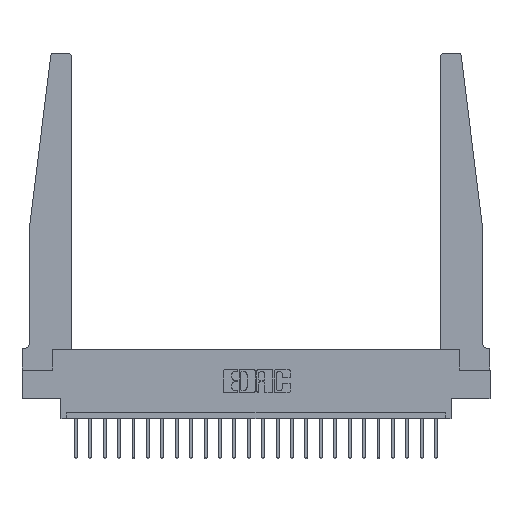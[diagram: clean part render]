
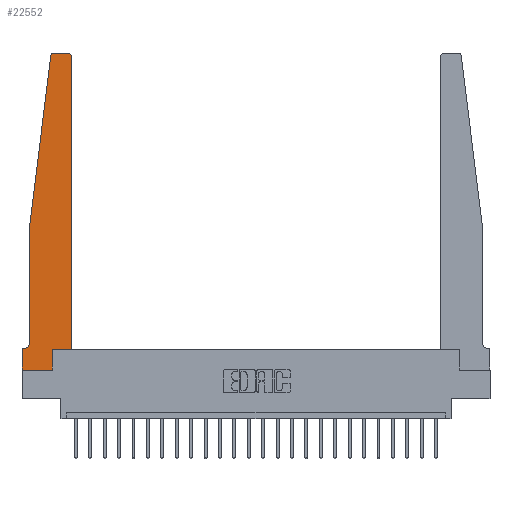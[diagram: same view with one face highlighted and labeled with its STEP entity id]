
A CAD part, top view. The second image highlights one B-rep face of the part: STEP entity #22552.
In plain terms, the highlighted planar face has unit normal (0, 0, 1).
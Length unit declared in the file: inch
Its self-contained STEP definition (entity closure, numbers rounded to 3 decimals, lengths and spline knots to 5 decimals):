
#285 = EDGE_CURVE ( 'NONE', #22686, #6802, #12120, .T. ) ;
#402 = VECTOR ( 'NONE', #20347, 39.37008 ) ;
#413 = VECTOR ( 'NONE', #7518, 39.37008 ) ;
#447 = EDGE_CURVE ( 'NONE', #7697, #12451, #21571, .T. ) ;
#527 = DIRECTION ( 'NONE',  ( 1., 0., 0. ) ) ;
#573 = CARTESIAN_POINT ( 'NONE',  ( 0.27653, 2.72, 0.37 ) ) ;
#1095 = CARTESIAN_POINT ( 'NONE',  ( 0.395, 2.75, 0.37 ) ) ;
#1218 = ORIENTED_EDGE ( 'NONE', *, *, #285, .T. ) ;
#1324 = DIRECTION ( 'NONE',  ( 1., 0., 0. ) ) ;
#1494 = VECTOR ( 'NONE', #14600, 39.37008 ) ;
#1548 = ORIENTED_EDGE ( 'NONE', *, *, #16300, .T. ) ;
#1681 = VECTOR ( 'NONE', #527, 39.37008 ) ;
#2255 = EDGE_CURVE ( 'NONE', #6659, #21559, #16882, .T. ) ;
#2371 = LINE ( 'NONE', #20222, #413 ) ;
#2618 = CARTESIAN_POINT ( 'NONE',  ( 0., 0., 0.37 ) ) ;
#2656 = DIRECTION ( 'NONE',  ( 1., 0., 0. ) ) ;
#2702 = EDGE_CURVE ( 'NONE', #4808, #13198, #22303, .T. ) ;
#3081 = VECTOR ( 'NONE', #17840, 39.37008 ) ;
#3187 = CIRCLE ( 'NONE', #11213, 0.05 ) ;
#3387 = CARTESIAN_POINT ( 'NONE',  ( 0.065, 1.25, 0.37 ) ) ;
#3524 = CARTESIAN_POINT ( 'NONE',  ( 0.425, 0.18, 0.37 ) ) ;
#4113 = CARTESIAN_POINT ( 'NONE',  ( 0.27653, 2.75, 0.37 ) ) ;
#4461 = EDGE_CURVE ( 'NONE', #21559, #7697, #10409, .T. ) ;
#4534 = CARTESIAN_POINT ( 'NONE',  ( 0.065, 0.2375, 0.37 ) ) ;
#4808 = VERTEX_POINT ( 'NONE', #2618 ) ;
#4922 = DIRECTION ( 'NONE',  ( 0., 0., 1. ) ) ;
#5050 = CARTESIAN_POINT ( 'NONE',  ( 0.065, 1.25, 0.37 ) ) ;
#5217 = ORIENTED_EDGE ( 'NONE', *, *, #14563, .T. ) ;
#6231 = VECTOR ( 'NONE', #12369, 39.37008 ) ;
#6659 = VERTEX_POINT ( 'NONE', #4113 ) ;
#6802 = VERTEX_POINT ( 'NONE', #1095 ) ;
#7161 = VECTOR ( 'NONE', #18108, 39.37008 ) ;
#7312 = CARTESIAN_POINT ( 'NONE',  ( 0.25, 2.75, 0.37 ) ) ;
#7518 = DIRECTION ( 'NONE',  ( 0., -1., 0. ) ) ;
#7689 = CARTESIAN_POINT ( 'NONE',  ( 0.24675, 2.72367, 0.37 ) ) ;
#7697 = VERTEX_POINT ( 'NONE', #15278 ) ;
#7989 = EDGE_CURVE ( 'NONE', #20314, #22686, #8184, .T. ) ;
#8154 = VERTEX_POINT ( 'NONE', #12374 ) ;
#8184 = LINE ( 'NONE', #9977, #17672 ) ;
#8438 = EDGE_CURVE ( 'NONE', #15799, #20314, #17579, .T. ) ;
#8598 = ORIENTED_EDGE ( 'NONE', *, *, #11076, .T. ) ;
#9106 = LINE ( 'NONE', #7312, #1494 ) ;
#9227 = CARTESIAN_POINT ( 'NONE',  ( 0.2605, 0.18, 0.37 ) ) ;
#9370 = ORIENTED_EDGE ( 'NONE', *, *, #21333, .T. ) ;
#9977 = CARTESIAN_POINT ( 'NONE',  ( 0.425, 0.18, 0.37 ) ) ;
#10087 = AXIS2_PLACEMENT_3D ( 'NONE', #13994, #4922, #1324 ) ;
#10281 = FACE_OUTER_BOUND ( 'NONE', #11730, .T. ) ;
#10409 = LINE ( 'NONE', #5050, #3081 ) ;
#11076 = EDGE_CURVE ( 'NONE', #8154, #20688, #12907, .T. ) ;
#11213 = AXIS2_PLACEMENT_3D ( 'NONE', #12381, #15721, #21484 ) ;
#11665 = DIRECTION ( 'NONE',  ( 0., 1., 0. ) ) ;
#11730 = EDGE_LOOP ( 'NONE', ( #5217, #13563, #23077, #22666, #15132, #8598, #1548, #17033, #9370, #17275, #16809, #1218 ) ) ;
#11896 = LINE ( 'NONE', #17513, #6231 ) ;
#12120 = CIRCLE ( 'NONE', #17862, 0.03 ) ;
#12369 = DIRECTION ( 'NONE',  ( 0., 1., 0. ) ) ;
#12374 = CARTESIAN_POINT ( 'NONE',  ( 0.015, 0.1875, 0.37 ) ) ;
#12381 = CARTESIAN_POINT ( 'NONE',  ( 0.015, 0.2375, 0.37 ) ) ;
#12451 = VERTEX_POINT ( 'NONE', #4534 ) ;
#12907 = LINE ( 'NONE', #15055, #402 ) ;
#13198 = VERTEX_POINT ( 'NONE', #18263 ) ;
#13209 = CARTESIAN_POINT ( 'NONE',  ( 0., 0., 0.37 ) ) ;
#13418 = CARTESIAN_POINT ( 'NONE',  ( 0.425, 0.18, 0.37 ) ) ;
#13457 = DIRECTION ( 'NONE',  ( 0., 0., 1. ) ) ;
#13563 = ORIENTED_EDGE ( 'NONE', *, *, #2255, .T. ) ;
#13994 = CARTESIAN_POINT ( 'NONE',  ( 0., 0.1875, 0.37 ) ) ;
#14563 = EDGE_CURVE ( 'NONE', #6802, #6659, #9106, .T. ) ;
#14600 = DIRECTION ( 'NONE',  ( -1., 0., 0. ) ) ;
#14706 = CARTESIAN_POINT ( 'NONE',  ( 0.425, 2.72, 0.37 ) ) ;
#15055 = CARTESIAN_POINT ( 'NONE',  ( 0.065, 0.1875, 0.37 ) ) ;
#15132 = ORIENTED_EDGE ( 'NONE', *, *, #21652, .T. ) ;
#15278 = CARTESIAN_POINT ( 'NONE',  ( 0.065, 1.25, 0.37 ) ) ;
#15721 = DIRECTION ( 'NONE',  ( 0., 0., -1. ) ) ;
#15799 = VERTEX_POINT ( 'NONE', #9227 ) ;
#16300 = EDGE_CURVE ( 'NONE', #20688, #4808, #2371, .T. ) ;
#16809 = ORIENTED_EDGE ( 'NONE', *, *, #7989, .T. ) ;
#16882 = CIRCLE ( 'NONE', #23383, 0.03 ) ;
#17033 = ORIENTED_EDGE ( 'NONE', *, *, #2702, .T. ) ;
#17275 = ORIENTED_EDGE ( 'NONE', *, *, #8438, .T. ) ;
#17513 = CARTESIAN_POINT ( 'NONE',  ( 0.2605, 0.18, 0.37 ) ) ;
#17579 = LINE ( 'NONE', #13418, #1681 ) ;
#17672 = VECTOR ( 'NONE', #11665, 39.37008 ) ;
#17840 = DIRECTION ( 'NONE',  ( -0.122, -0.992, 0. ) ) ;
#17862 = AXIS2_PLACEMENT_3D ( 'NONE', #22643, #19424, #2656 ) ;
#18108 = DIRECTION ( 'NONE',  ( 0., -1., 0. ) ) ;
#18263 = CARTESIAN_POINT ( 'NONE',  ( 0.2605, 0., 0.37 ) ) ;
#18640 = DIRECTION ( 'NONE',  ( 1., 0., 0. ) ) ;
#19424 = DIRECTION ( 'NONE',  ( 0., 0., 1. ) ) ;
#19620 = VECTOR ( 'NONE', #22425, 39.37008 ) ;
#19647 = CARTESIAN_POINT ( 'NONE',  ( 0., 0.1875, 0.37 ) ) ;
#20222 = CARTESIAN_POINT ( 'NONE',  ( 0., 0., 0.37 ) ) ;
#20314 = VERTEX_POINT ( 'NONE', #3524 ) ;
#20347 = DIRECTION ( 'NONE',  ( -1., 0., 0. ) ) ;
#20688 = VERTEX_POINT ( 'NONE', #19647 ) ;
#20943 = PLANE ( 'NONE',  #10087 ) ;
#21333 = EDGE_CURVE ( 'NONE', #13198, #15799, #11896, .T. ) ;
#21484 = DIRECTION ( 'NONE',  ( -1., 0., 0. ) ) ;
#21559 = VERTEX_POINT ( 'NONE', #7689 ) ;
#21571 = LINE ( 'NONE', #3387, #7161 ) ;
#21652 = EDGE_CURVE ( 'NONE', #12451, #8154, #3187, .T. ) ;
#22303 = LINE ( 'NONE', #13209, #19620 ) ;
#22425 = DIRECTION ( 'NONE',  ( 1., 0., 0. ) ) ;
#22552 = ADVANCED_FACE ( 'NONE', ( #10281 ), #20943, .T. ) ;
#22643 = CARTESIAN_POINT ( 'NONE',  ( 0.395, 2.72, 0.37 ) ) ;
#22666 = ORIENTED_EDGE ( 'NONE', *, *, #447, .T. ) ;
#22686 = VERTEX_POINT ( 'NONE', #14706 ) ;
#23077 = ORIENTED_EDGE ( 'NONE', *, *, #4461, .T. ) ;
#23383 = AXIS2_PLACEMENT_3D ( 'NONE', #573, #13457, #18640 ) ;
